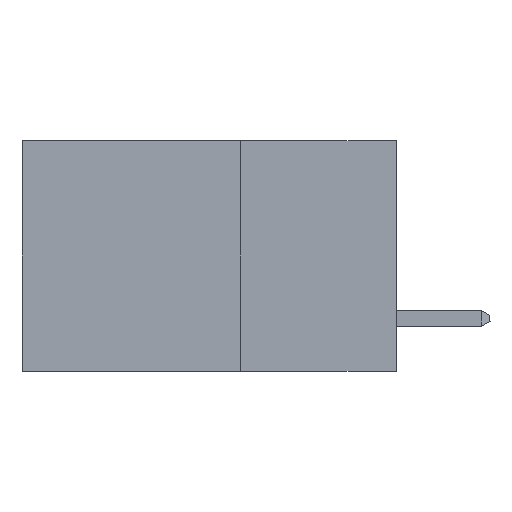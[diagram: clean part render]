
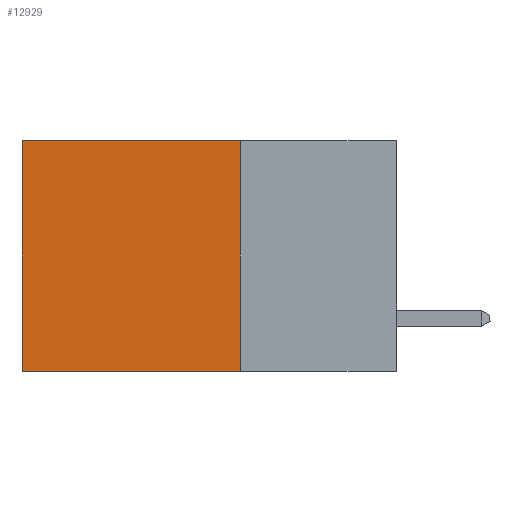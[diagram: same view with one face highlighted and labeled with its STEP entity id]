
A CAD part, left-side view. The second image highlights one B-rep face of the part: STEP entity #12929.
In plain terms, the highlighted planar face has unit normal (-1, 0, 0).
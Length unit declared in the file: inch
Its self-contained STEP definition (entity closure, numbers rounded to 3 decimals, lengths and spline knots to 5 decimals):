
#57 = ORIENTED_EDGE ( 'NONE', *, *, #12249, .T. ) ;
#762 = DIRECTION ( 'NONE',  ( 0., 1., 0. ) ) ;
#820 = CARTESIAN_POINT ( 'NONE',  ( 0.298, 0.25, -0.37 ) ) ;
#923 = VERTEX_POINT ( 'NONE', #1532 ) ;
#1486 = VECTOR ( 'NONE', #2078, 39.37008 ) ;
#1532 = CARTESIAN_POINT ( 'NONE',  ( 0.298, 0.6, -0.37 ) ) ;
#2078 = DIRECTION ( 'NONE',  ( 0., 0., -1. ) ) ;
#3084 = ORIENTED_EDGE ( 'NONE', *, *, #11612, .F. ) ;
#3120 = DIRECTION ( 'NONE',  ( 0., 0., -1. ) ) ;
#3471 = DIRECTION ( 'NONE',  ( 1., 0., 0. ) ) ;
#4240 = LINE ( 'NONE', #8397, #1486 ) ;
#4488 = EDGE_LOOP ( 'NONE', ( #5317, #3084, #9200, #57 ) ) ;
#4672 = CARTESIAN_POINT ( 'NONE',  ( 0.298, 0.25, 0. ) ) ;
#4922 = EDGE_CURVE ( 'NONE', #6367, #923, #7816, .T. ) ;
#4953 = CARTESIAN_POINT ( 'NONE',  ( 0.298, 0.25, 0. ) ) ;
#5317 = ORIENTED_EDGE ( 'NONE', *, *, #4922, .T. ) ;
#5982 = CARTESIAN_POINT ( 'NONE',  ( 0.298, 0.25, -0.37 ) ) ;
#6302 = CARTESIAN_POINT ( 'NONE',  ( 0.298, 0.25, 0. ) ) ;
#6367 = VERTEX_POINT ( 'NONE', #10465 ) ;
#7294 = VECTOR ( 'NONE', #10098, 39.37008 ) ;
#7326 = VECTOR ( 'NONE', #3120, 39.37008 ) ;
#7800 = PLANE ( 'NONE',  #12806 ) ;
#7816 = LINE ( 'NONE', #9341, #7326 ) ;
#7937 = LINE ( 'NONE', #5982, #11822 ) ;
#7976 = VERTEX_POINT ( 'NONE', #820 ) ;
#8397 = CARTESIAN_POINT ( 'NONE',  ( 0.298, 0.25, 0. ) ) ;
#8552 = FACE_OUTER_BOUND ( 'NONE', #4488, .T. ) ;
#9200 = ORIENTED_EDGE ( 'NONE', *, *, #9824, .F. ) ;
#9341 = CARTESIAN_POINT ( 'NONE',  ( 0.298, 0.6, 0. ) ) ;
#9824 = EDGE_CURVE ( 'NONE', #10444, #7976, #4240, .T. ) ;
#10098 = DIRECTION ( 'NONE',  ( 0., 1., 0. ) ) ;
#10444 = VERTEX_POINT ( 'NONE', #6302 ) ;
#10465 = CARTESIAN_POINT ( 'NONE',  ( 0.298, 0.6, 0. ) ) ;
#11344 = LINE ( 'NONE', #4953, #7294 ) ;
#11612 = EDGE_CURVE ( 'NONE', #7976, #923, #7937, .T. ) ;
#11822 = VECTOR ( 'NONE', #762, 39.37008 ) ;
#11863 = DIRECTION ( 'NONE',  ( 0., 0., -1. ) ) ;
#12249 = EDGE_CURVE ( 'NONE', #10444, #6367, #11344, .T. ) ;
#12806 = AXIS2_PLACEMENT_3D ( 'NONE', #4672, #3471, #11863 ) ;
#12929 = ADVANCED_FACE ( 'NONE', ( #8552 ), #7800, .F. ) ;
